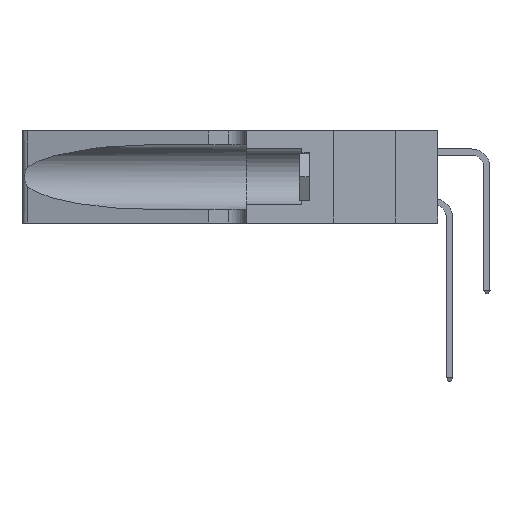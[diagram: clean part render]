
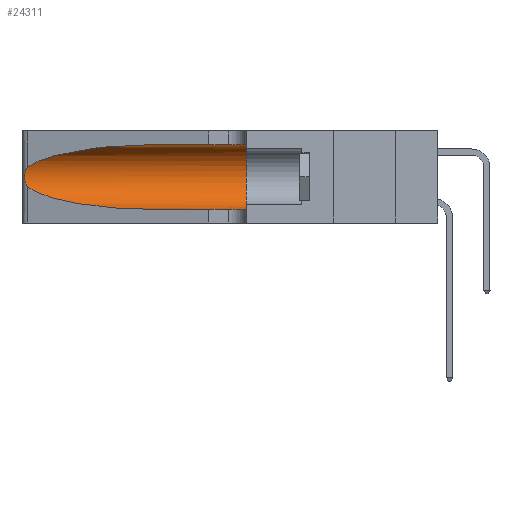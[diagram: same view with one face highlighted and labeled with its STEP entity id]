
A CAD part, left-side view. The second image highlights one B-rep face of the part: STEP entity #24311.
In plain terms, the highlighted cylindrical face has radius 3.308 mm (diameter 6.617 mm), a partial arc.
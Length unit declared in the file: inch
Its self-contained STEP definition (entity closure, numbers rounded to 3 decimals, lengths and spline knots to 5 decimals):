
#128 = CYLINDRICAL_SURFACE ( 'NONE', #27656, 0.13025 ) ;
#134 = CARTESIAN_POINT ( 'NONE',  ( 0.1305, 0.35, 0.31525 ) ) ;
#269 = CARTESIAN_POINT ( 'NONE',  ( 0.25487, 1.22718, 0.14631 ) ) ;
#1831 = CARTESIAN_POINT ( 'NONE',  ( 0.2373, 1.15595, 0.28018 ) ) ;
#1917 = CARTESIAN_POINT ( 'NONE',  ( 0.1305, 1.61858, 0.31525 ) ) ;
#2428 = EDGE_LOOP ( 'NONE', ( #11013, #8449, #2666, #12404, #19045, #19102 ) ) ;
#2636 = EDGE_CURVE ( 'NONE', #25665, #2716, #5442, .T. ) ;
#2666 = ORIENTED_EDGE ( 'NONE', *, *, #13001, .T. ) ;
#2716 = VERTEX_POINT ( 'NONE', #134 ) ;
#2767 = CARTESIAN_POINT ( 'NONE',  ( 0.18966, 0.96281, 0.05475 ) ) ;
#3879 = CARTESIAN_POINT ( 'NONE',  ( 0.26075, 1.23896, 0.178 ) ) ;
#4879 = AXIS2_PLACEMENT_3D ( 'NONE', #15629, #22613, #6625 ) ;
#5442 = LINE ( 'NONE', #1917, #13033 ) ;
#5976 = CARTESIAN_POINT ( 'NONE',  ( 0.25487, 1.22718, 0.14631 ) ) ;
#6203 = CARTESIAN_POINT ( 'NONE',  ( 0.26017, 1.23833, 0.17102 ) ) ;
#6302 = CARTESIAN_POINT ( 'NONE',  ( 0.26018, 1.23835, 0.19895 ) ) ;
#6460 = CARTESIAN_POINT ( 'NONE',  ( 0.25487, 1.22718, 0.22369 ) ) ;
#6496 = CARTESIAN_POINT ( 'NONE',  ( 0.26075, 1.23896, 0.19203 ) ) ;
#6625 = DIRECTION ( 'NONE',  ( 0., 0., 1. ) ) ;
#6920 = VERTEX_POINT ( 'NONE', #9789 ) ;
#7313 =( BOUNDED_CURVE ( )  B_SPLINE_CURVE ( 3, ( #269, #12134, #2767, #14477 ),
 .UNSPECIFIED., .F., .T. ) 
 B_SPLINE_CURVE_WITH_KNOTS ( ( 4, 4 ),
 ( 3.44316, 4.71239 ),
 .UNSPECIFIED. ) 
 CURVE ( )  GEOMETRIC_REPRESENTATION_ITEM ( )  RATIONAL_B_SPLINE_CURVE ( ( 1., 0.87, 0.87, 1. ) ) 
 REPRESENTATION_ITEM ( '' )  );
#7345 = DIRECTION ( 'NONE',  ( 0., 0., -1. ) ) ;
#8449 = ORIENTED_EDGE ( 'NONE', *, *, #12645, .T. ) ;
#8518 = CARTESIAN_POINT ( 'NONE',  ( 0.25639, 1.23186, 0.15144 ) ) ;
#8622 = CARTESIAN_POINT ( 'NONE',  ( 0.25555, 1.22993, 0.14849 ) ) ;
#8918 = CARTESIAN_POINT ( 'NONE',  ( 0.25487, 1.22718, 0.14631 ) ) ;
#9789 = CARTESIAN_POINT ( 'NONE',  ( 0.1305, 0.72297, 0.05475 ) ) ;
#10477 = B_SPLINE_CURVE_WITH_KNOTS ( 'NONE', 3,
 ( #15780, #24813, #20015, #29525, #22388, #6302, #6496, #3879, #6203, #17875, #17979, #8518, #8622, #8918 ),
 .UNSPECIFIED., .F., .F.,
 ( 4, 2, 2, 2, 2, 2, 4 ),
 ( 0., 0.00027, 0.00053, 0.00107, 0.0016, 0.00187, 0.00214 ),
 .UNSPECIFIED. ) ;
#11013 = ORIENTED_EDGE ( 'NONE', *, *, #13468, .T. ) ;
#11088 = LINE ( 'NONE', #12918, #13276 ) ;
#11689 = CARTESIAN_POINT ( 'NONE',  ( 0.25487, 1.22718, 0.22369 ) ) ;
#12134 = CARTESIAN_POINT ( 'NONE',  ( 0.2373, 1.15595, 0.08982 ) ) ;
#12404 = ORIENTED_EDGE ( 'NONE', *, *, #16686, .T. ) ;
#12645 = EDGE_CURVE ( 'NONE', #13521, #13257, #10477, .T. ) ;
#12918 = CARTESIAN_POINT ( 'NONE',  ( 0.1305, 1.61858, 0.05475 ) ) ;
#13001 = EDGE_CURVE ( 'NONE', #13257, #6920, #7313, .T. ) ;
#13033 = VECTOR ( 'NONE', #15834, 39.37008 ) ;
#13257 = VERTEX_POINT ( 'NONE', #5976 ) ;
#13276 = VECTOR ( 'NONE', #29274, 39.37008 ) ;
#13335 = CARTESIAN_POINT ( 'NONE',  ( 0.1305, 0.72297, 0.31525 ) ) ;
#13468 = EDGE_CURVE ( 'NONE', #25665, #13521, #28164, .T. ) ;
#13521 = VERTEX_POINT ( 'NONE', #11689 ) ;
#14477 = CARTESIAN_POINT ( 'NONE',  ( 0.1305, 0.72297, 0.05475 ) ) ;
#14918 = FACE_OUTER_BOUND ( 'NONE', #2428, .T. ) ;
#15629 = CARTESIAN_POINT ( 'NONE',  ( 0.1305, 0.35, 0.185 ) ) ;
#15657 = CARTESIAN_POINT ( 'NONE',  ( 0.18966, 0.96281, 0.31525 ) ) ;
#15780 = CARTESIAN_POINT ( 'NONE',  ( 0.25487, 1.22718, 0.22369 ) ) ;
#15834 = DIRECTION ( 'NONE',  ( 0., -1., 0. ) ) ;
#16542 = DIRECTION ( 'NONE',  ( 0., -1., 0. ) ) ;
#16686 = EDGE_CURVE ( 'NONE', #6920, #23485, #11088, .T. ) ;
#17642 = CIRCLE ( 'NONE', #4879, 0.13025 ) ;
#17875 = CARTESIAN_POINT ( 'NONE',  ( 0.25856, 1.23593, 0.16098 ) ) ;
#17979 = CARTESIAN_POINT ( 'NONE',  ( 0.25789, 1.23486, 0.15765 ) ) ;
#18362 = CARTESIAN_POINT ( 'NONE',  ( 0.1305, 0.72297, 0.31525 ) ) ;
#19045 = ORIENTED_EDGE ( 'NONE', *, *, #19910, .F. ) ;
#19102 = ORIENTED_EDGE ( 'NONE', *, *, #2636, .F. ) ;
#19264 = CARTESIAN_POINT ( 'NONE',  ( 0.1305, 0.35, 0.05475 ) ) ;
#19910 = EDGE_CURVE ( 'NONE', #2716, #23485, #17642, .T. ) ;
#20015 = CARTESIAN_POINT ( 'NONE',  ( 0.25639, 1.23184, 0.21858 ) ) ;
#22388 = CARTESIAN_POINT ( 'NONE',  ( 0.25854, 1.2359, 0.20912 ) ) ;
#22613 = DIRECTION ( 'NONE',  ( 0., 1., 0. ) ) ;
#23485 = VERTEX_POINT ( 'NONE', #19264 ) ;
#24311 = ADVANCED_FACE ( 'NONE', ( #14918 ), #128, .F. ) ;
#24813 = CARTESIAN_POINT ( 'NONE',  ( 0.25555, 1.22994, 0.2215 ) ) ;
#25370 = CARTESIAN_POINT ( 'NONE',  ( 0.1305, 1.61858, 0.185 ) ) ;
#25665 = VERTEX_POINT ( 'NONE', #18362 ) ;
#27656 = AXIS2_PLACEMENT_3D ( 'NONE', #25370, #16542, #7345 ) ;
#28164 =( BOUNDED_CURVE ( )  B_SPLINE_CURVE ( 3, ( #13335, #15657, #1831, #6460 ),
 .UNSPECIFIED., .F., .F. ) 
 B_SPLINE_CURVE_WITH_KNOTS ( ( 4, 4 ),
 ( 1.5708, 2.84003 ),
 .UNSPECIFIED. ) 
 CURVE ( )  GEOMETRIC_REPRESENTATION_ITEM ( )  RATIONAL_B_SPLINE_CURVE ( ( 1., 0.87, 0.87, 1. ) ) 
 REPRESENTATION_ITEM ( '' )  );
#29274 = DIRECTION ( 'NONE',  ( 0., -1., 0. ) ) ;
#29525 = CARTESIAN_POINT ( 'NONE',  ( 0.25787, 1.23484, 0.2124 ) ) ;
